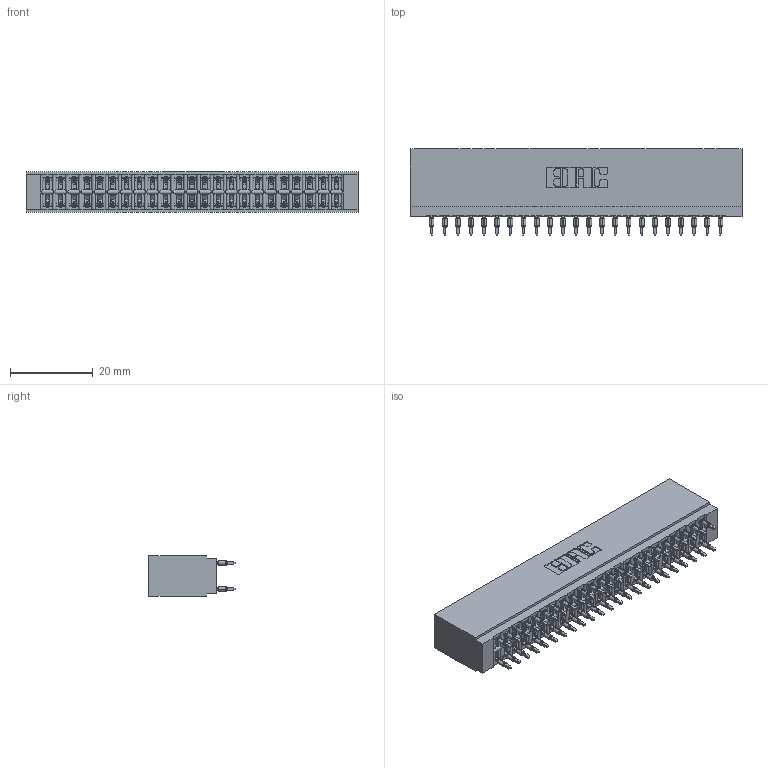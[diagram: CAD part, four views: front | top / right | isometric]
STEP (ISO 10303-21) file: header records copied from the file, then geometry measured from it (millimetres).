
FILE_DESCRIPTION (( 'STEP AP203' ), '1' );
FILE_NAME ('746-046-560-201.STEP', '2020-09-16T23:53:09', ( '' ), ( '' ), 'SwSTEP 2.0', 'SolidWorks 2020', '' );
FILE_SCHEMA (( 'CONFIG_CONTROL_DESIGN' ));
Length unit declared in the file: inch
Products named in the file (3): 746-046-560-201; 746-292-001_560; 746 Part_.515 Slot Depth - 01
Assembly tree (47 placements, depth 2):
  746-046-560-201
    746 Part_.515 Slot Depth - 01
    746-292-001_560  x46
Bounding box: 80.26 x 20.82 x 9.91 mm (x, y, z)
Volume: 8901.5 mm3; surface area: 14777.3 mm2
Topology: 47 solids, 47 shells, 4444 faces, 12361 edges, 7926 vertices
Faces by surface type: plane 2217, cylinder 1031, bspline 920, torus 276
Entity records: 38368 total; most frequent: CARTESIAN_POINT 7789, ORIENTED_EDGE 6542, DIRECTION 5501, EDGE_CURVE 3271, LINE 2849, VECTOR 2849, VERTEX_POINT 2166, AXIS2_PLACEMENT_3D 1326
